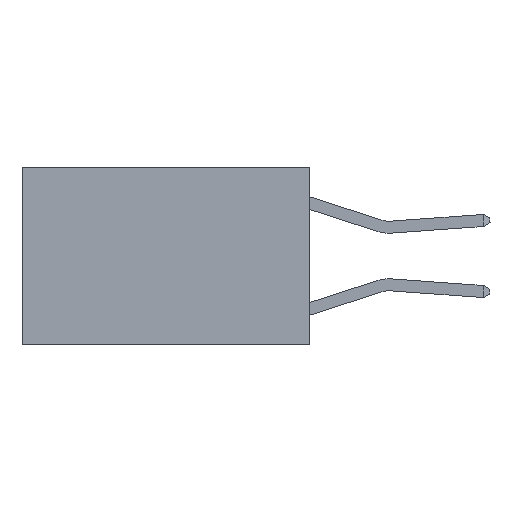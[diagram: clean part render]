
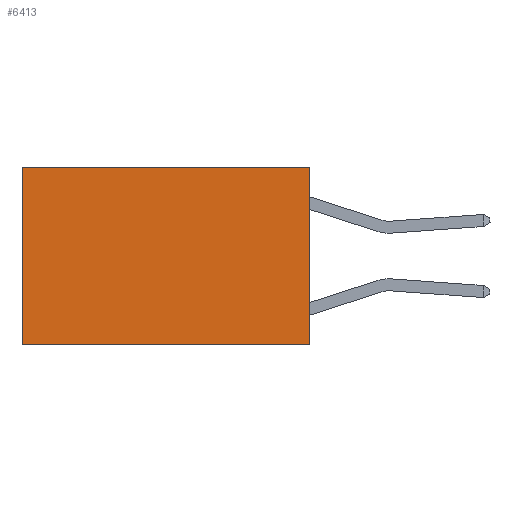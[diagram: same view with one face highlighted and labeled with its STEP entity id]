
A CAD part, left-side view. The second image highlights one B-rep face of the part: STEP entity #6413.
In plain terms, the highlighted planar face has unit normal (-1, 0, 0).
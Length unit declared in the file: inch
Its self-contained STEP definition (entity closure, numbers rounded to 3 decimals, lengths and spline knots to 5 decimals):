
#360 = DIRECTION ( 'NONE',  ( 0., 0., -1. ) ) ;
#474 = ORIENTED_EDGE ( 'NONE', *, *, #784, .T. ) ;
#784 = EDGE_CURVE ( 'NONE', #9937, #4135, #4481, .T. ) ;
#978 = CARTESIAN_POINT ( 'NONE',  ( 0.2625, 0.6, 0. ) ) ;
#1052 = VERTEX_POINT ( 'NONE', #9363 ) ;
#1590 = CARTESIAN_POINT ( 'NONE',  ( 0.2625, 0., 0. ) ) ;
#2126 = CARTESIAN_POINT ( 'NONE',  ( 0.2625, 0.6, 0. ) ) ;
#2168 = ORIENTED_EDGE ( 'NONE', *, *, #6781, .T. ) ;
#2171 = LINE ( 'NONE', #10241, #6870 ) ;
#3317 = ORIENTED_EDGE ( 'NONE', *, *, #9535, .F. ) ;
#3418 = DIRECTION ( 'NONE',  ( 0., 0., -1. ) ) ;
#3584 = CARTESIAN_POINT ( 'NONE',  ( 0.2625, 0., -0.37 ) ) ;
#4135 = VERTEX_POINT ( 'NONE', #4275 ) ;
#4187 = ORIENTED_EDGE ( 'NONE', *, *, #9298, .F. ) ;
#4275 = CARTESIAN_POINT ( 'NONE',  ( 0.2625, 0.6, -0.37 ) ) ;
#4318 = DIRECTION ( 'NONE',  ( 0., 1., 0. ) ) ;
#4481 = LINE ( 'NONE', #978, #8894 ) ;
#4504 = DIRECTION ( 'NONE',  ( 0., 1., 0. ) ) ;
#4520 = VECTOR ( 'NONE', #4318, 39.37008 ) ;
#4805 = LINE ( 'NONE', #7053, #4520 ) ;
#5461 = AXIS2_PLACEMENT_3D ( 'NONE', #1590, #10796, #6001 ) ;
#6001 = DIRECTION ( 'NONE',  ( 0., 0., -1. ) ) ;
#6272 = LINE ( 'NONE', #3584, #9892 ) ;
#6413 = ADVANCED_FACE ( 'NONE', ( #8452 ), #10099, .F. ) ;
#6781 = EDGE_CURVE ( 'NONE', #1052, #9937, #4805, .T. ) ;
#6870 = VECTOR ( 'NONE', #3418, 39.37008 ) ;
#7053 = CARTESIAN_POINT ( 'NONE',  ( 0.2625, 0., 0. ) ) ;
#8452 = FACE_OUTER_BOUND ( 'NONE', #10508, .T. ) ;
#8894 = VECTOR ( 'NONE', #360, 39.37008 ) ;
#9298 = EDGE_CURVE ( 'NONE', #1052, #9494, #2171, .T. ) ;
#9363 = CARTESIAN_POINT ( 'NONE',  ( 0.2625, 0., 0. ) ) ;
#9494 = VERTEX_POINT ( 'NONE', #9586 ) ;
#9535 = EDGE_CURVE ( 'NONE', #9494, #4135, #6272, .T. ) ;
#9586 = CARTESIAN_POINT ( 'NONE',  ( 0.2625, 0., -0.37 ) ) ;
#9892 = VECTOR ( 'NONE', #4504, 39.37008 ) ;
#9937 = VERTEX_POINT ( 'NONE', #2126 ) ;
#10099 = PLANE ( 'NONE',  #5461 ) ;
#10241 = CARTESIAN_POINT ( 'NONE',  ( 0.2625, 0., 0. ) ) ;
#10508 = EDGE_LOOP ( 'NONE', ( #474, #3317, #4187, #2168 ) ) ;
#10796 = DIRECTION ( 'NONE',  ( 1., 0., 0. ) ) ;
